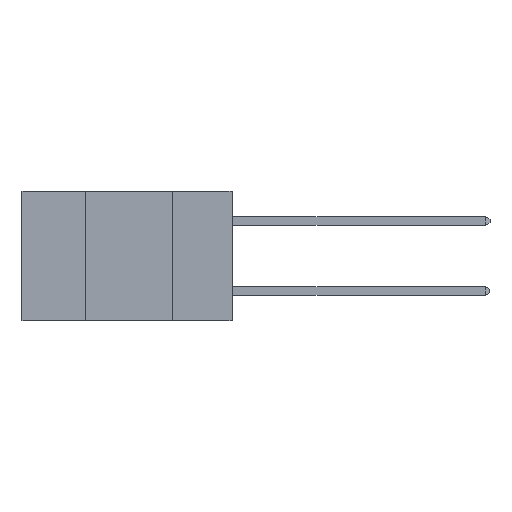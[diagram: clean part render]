
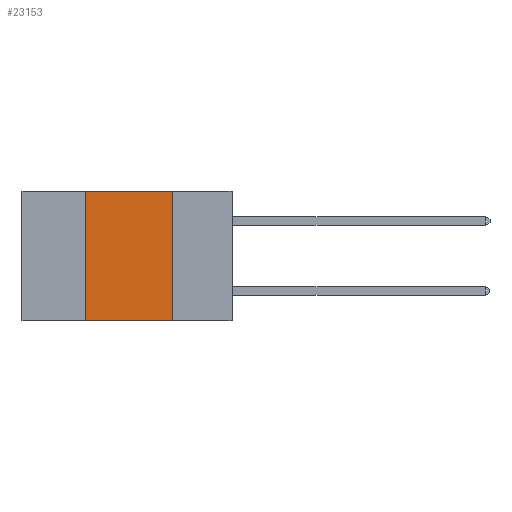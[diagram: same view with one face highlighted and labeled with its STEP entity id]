
A CAD part, left-side view. The second image highlights one B-rep face of the part: STEP entity #23153.
In plain terms, the highlighted planar face has unit normal (-1, 0, 0).
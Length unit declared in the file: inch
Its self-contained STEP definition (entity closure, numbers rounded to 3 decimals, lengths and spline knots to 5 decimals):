
#525 = VECTOR ( 'NONE', #4226, 39.37008 ) ;
#1712 = EDGE_LOOP ( 'NONE', ( #18001, #18018, #18494, #19182 ) ) ;
#2024 = LINE ( 'NONE', #14669, #21037 ) ;
#3081 = VERTEX_POINT ( 'NONE', #12129 ) ;
#3189 = CARTESIAN_POINT ( 'NONE',  ( 0., 0.6, 0. ) ) ;
#4226 = DIRECTION ( 'NONE',  ( 0., 0., 1. ) ) ;
#4945 = PLANE ( 'NONE',  #9702 ) ;
#6961 = DIRECTION ( 'NONE',  ( 1., 0., 0. ) ) ;
#7791 = VERTEX_POINT ( 'NONE', #8724 ) ;
#8434 = VERTEX_POINT ( 'NONE', #12767 ) ;
#8724 = CARTESIAN_POINT ( 'NONE',  ( 0., 0.42, 0. ) ) ;
#9702 = AXIS2_PLACEMENT_3D ( 'NONE', #12459, #6961, #19576 ) ;
#10658 = LINE ( 'NONE', #15329, #525 ) ;
#11472 = LINE ( 'NONE', #3189, #19243 ) ;
#12065 = CARTESIAN_POINT ( 'NONE',  ( 0., 0.6, -0.37 ) ) ;
#12129 = CARTESIAN_POINT ( 'NONE',  ( 0., 0.17, -0.37 ) ) ;
#12459 = CARTESIAN_POINT ( 'NONE',  ( 0., 0.6, 0. ) ) ;
#12571 = EDGE_CURVE ( 'NONE', #21267, #3081, #20803, .T. ) ;
#12767 = CARTESIAN_POINT ( 'NONE',  ( 0., 0.17, 0. ) ) ;
#13743 = EDGE_CURVE ( 'NONE', #21267, #7791, #10658, .T. ) ;
#13808 = VECTOR ( 'NONE', #13813, 39.37008 ) ;
#13813 = DIRECTION ( 'NONE',  ( 0., -1., 0. ) ) ;
#13902 = FACE_OUTER_BOUND ( 'NONE', #1712, .T. ) ;
#14669 = CARTESIAN_POINT ( 'NONE',  ( 0., 0.17, 0. ) ) ;
#15329 = CARTESIAN_POINT ( 'NONE',  ( 0., 0.42, 0. ) ) ;
#16430 = DIRECTION ( 'NONE',  ( 0., 0., -1. ) ) ;
#18001 = ORIENTED_EDGE ( 'NONE', *, *, #23300, .F. ) ;
#18018 = ORIENTED_EDGE ( 'NONE', *, *, #22264, .F. ) ;
#18494 = ORIENTED_EDGE ( 'NONE', *, *, #13743, .F. ) ;
#19182 = ORIENTED_EDGE ( 'NONE', *, *, #12571, .T. ) ;
#19243 = VECTOR ( 'NONE', #23340, 39.37008 ) ;
#19576 = DIRECTION ( 'NONE',  ( 0., 0., -1. ) ) ;
#20803 = LINE ( 'NONE', #12065, #13808 ) ;
#21037 = VECTOR ( 'NONE', #16430, 39.37008 ) ;
#21267 = VERTEX_POINT ( 'NONE', #22310 ) ;
#22264 = EDGE_CURVE ( 'NONE', #7791, #8434, #11472, .T. ) ;
#22310 = CARTESIAN_POINT ( 'NONE',  ( 0., 0.42, -0.37 ) ) ;
#23153 = ADVANCED_FACE ( 'NONE', ( #13902 ), #4945, .F. ) ;
#23300 = EDGE_CURVE ( 'NONE', #8434, #3081, #2024, .T. ) ;
#23340 = DIRECTION ( 'NONE',  ( 0., -1., 0. ) ) ;
